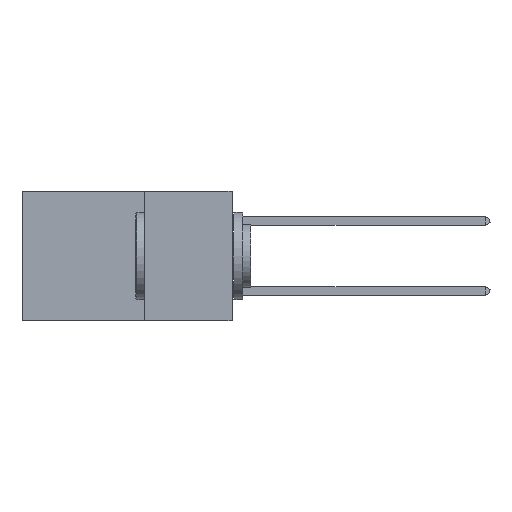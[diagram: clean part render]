
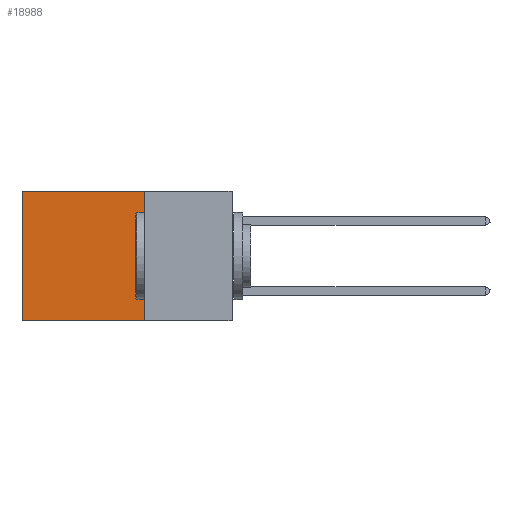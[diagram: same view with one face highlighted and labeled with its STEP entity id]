
A CAD part, left-side view. The second image highlights one B-rep face of the part: STEP entity #18988.
In plain terms, the highlighted planar face has unit normal (-1, 0, 0).
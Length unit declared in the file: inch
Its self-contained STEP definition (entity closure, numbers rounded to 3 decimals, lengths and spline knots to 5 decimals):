
#14 = CARTESIAN_POINT ( 'NONE',  ( 0.2875, 0.25, 0. ) ) ;
#306 = VECTOR ( 'NONE', #43918, 39.37008 ) ;
#1868 = VERTEX_POINT ( 'NONE', #14 ) ;
#2304 = ORIENTED_EDGE ( 'NONE', *, *, #6031, .F. ) ;
#5816 = CARTESIAN_POINT ( 'NONE',  ( 0.2875, 0.6, -0.37 ) ) ;
#5975 = AXIS2_PLACEMENT_3D ( 'NONE', #32933, #43864, #36616 ) ;
#6031 = EDGE_CURVE ( 'NONE', #1868, #9294, #36492, .T. ) ;
#7156 = LINE ( 'NONE', #29952, #306 ) ;
#9294 = VERTEX_POINT ( 'NONE', #38607 ) ;
#9338 = CARTESIAN_POINT ( 'NONE',  ( 0.2875, 0.6, 0. ) ) ;
#9797 = EDGE_CURVE ( 'NONE', #40457, #38482, #7156, .T. ) ;
#9800 = EDGE_CURVE ( 'NONE', #1868, #40457, #27102, .T. ) ;
#12435 = EDGE_LOOP ( 'NONE', ( #25894, #40877, #2304, #16804 ) ) ;
#14520 = PLANE ( 'NONE',  #5975 ) ;
#15740 = DIRECTION ( 'NONE',  ( 0., 1., 0. ) ) ;
#16804 = ORIENTED_EDGE ( 'NONE', *, *, #9800, .T. ) ;
#17759 = VECTOR ( 'NONE', #24898, 39.37008 ) ;
#18988 = ADVANCED_FACE ( 'NONE', ( #26189 ), #14520, .F. ) ;
#22216 = CARTESIAN_POINT ( 'NONE',  ( 0.2875, 0.25, 0. ) ) ;
#24898 = DIRECTION ( 'NONE',  ( 0., 0., -1. ) ) ;
#25894 = ORIENTED_EDGE ( 'NONE', *, *, #9797, .T. ) ;
#26189 = FACE_OUTER_BOUND ( 'NONE', #12435, .T. ) ;
#27102 = LINE ( 'NONE', #22216, #35623 ) ;
#28050 = VECTOR ( 'NONE', #15740, 39.37008 ) ;
#29952 = CARTESIAN_POINT ( 'NONE',  ( 0.2875, 0.6, 0. ) ) ;
#30474 = CARTESIAN_POINT ( 'NONE',  ( 0.2875, 0.25, -0.37 ) ) ;
#32017 = CARTESIAN_POINT ( 'NONE',  ( 0.2875, 0.25, 0. ) ) ;
#32933 = CARTESIAN_POINT ( 'NONE',  ( 0.2875, 0.25, 0. ) ) ;
#34415 = EDGE_CURVE ( 'NONE', #9294, #38482, #41671, .T. ) ;
#35623 = VECTOR ( 'NONE', #40297, 39.37008 ) ;
#36492 = LINE ( 'NONE', #32017, #17759 ) ;
#36616 = DIRECTION ( 'NONE',  ( 0., 0., -1. ) ) ;
#38482 = VERTEX_POINT ( 'NONE', #5816 ) ;
#38607 = CARTESIAN_POINT ( 'NONE',  ( 0.2875, 0.25, -0.37 ) ) ;
#40297 = DIRECTION ( 'NONE',  ( 0., 1., 0. ) ) ;
#40457 = VERTEX_POINT ( 'NONE', #9338 ) ;
#40877 = ORIENTED_EDGE ( 'NONE', *, *, #34415, .F. ) ;
#41671 = LINE ( 'NONE', #30474, #28050 ) ;
#43864 = DIRECTION ( 'NONE',  ( 1., 0., 0. ) ) ;
#43918 = DIRECTION ( 'NONE',  ( 0., 0., -1. ) ) ;
